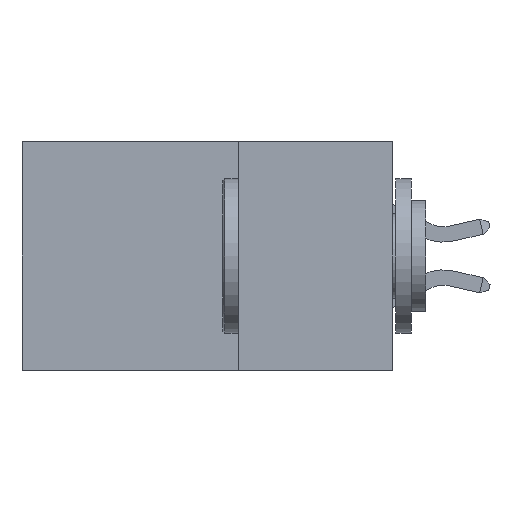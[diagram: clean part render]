
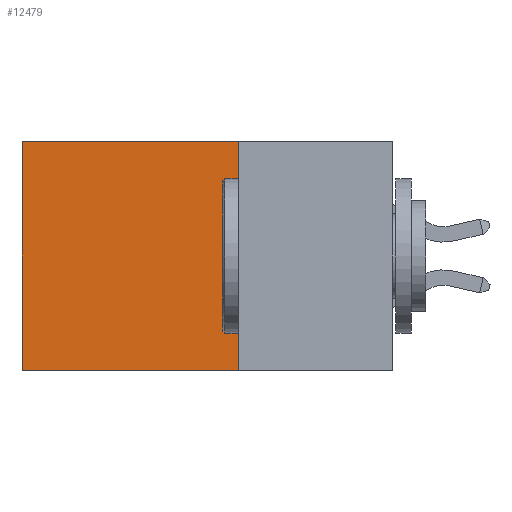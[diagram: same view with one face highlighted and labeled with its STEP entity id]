
A CAD part, left-side view. The second image highlights one B-rep face of the part: STEP entity #12479.
In plain terms, the highlighted planar face has unit normal (-1, 0, 0).
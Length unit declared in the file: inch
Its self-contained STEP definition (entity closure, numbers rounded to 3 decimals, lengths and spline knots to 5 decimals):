
#1397 = CARTESIAN_POINT ( 'NONE',  ( 0.2875, 0.6, 0. ) ) ;
#2869 = EDGE_CURVE ( 'NONE', #35021, #25414, #23550, .T. ) ;
#4264 = EDGE_CURVE ( 'NONE', #35021, #15242, #15848, .T. ) ;
#4286 = VECTOR ( 'NONE', #32611, 39.37008 ) ;
#5273 = CARTESIAN_POINT ( 'NONE',  ( 0.2875, 0.25, 0. ) ) ;
#5364 = DIRECTION ( 'NONE',  ( 0., 0., -1. ) ) ;
#6828 = CARTESIAN_POINT ( 'NONE',  ( 0.2875, 0.25, 0. ) ) ;
#7261 = DIRECTION ( 'NONE',  ( 0., 0., -1. ) ) ;
#8185 = CARTESIAN_POINT ( 'NONE',  ( 0.2875, 0.25, 0. ) ) ;
#8508 = DIRECTION ( 'NONE',  ( 0., 1., 0. ) ) ;
#10501 = VERTEX_POINT ( 'NONE', #10815 ) ;
#10815 = CARTESIAN_POINT ( 'NONE',  ( 0.2875, 0.6, -0.37 ) ) ;
#11684 = DIRECTION ( 'NONE',  ( 1., 0., 0. ) ) ;
#12479 = ADVANCED_FACE ( 'NONE', ( #28546 ), #18014, .F. ) ;
#15242 = VERTEX_POINT ( 'NONE', #37734 ) ;
#15775 = CARTESIAN_POINT ( 'NONE',  ( 0.2875, 0.25, 0. ) ) ;
#15848 = LINE ( 'NONE', #15775, #37010 ) ;
#16055 = EDGE_CURVE ( 'NONE', #25414, #10501, #39386, .T. ) ;
#18014 = PLANE ( 'NONE',  #30349 ) ;
#18202 = CARTESIAN_POINT ( 'NONE',  ( 0.2875, 0.6, 0. ) ) ;
#19300 = DIRECTION ( 'NONE',  ( 0., 0., -1. ) ) ;
#21228 = VECTOR ( 'NONE', #7261, 39.37008 ) ;
#23550 = LINE ( 'NONE', #5273, #28610 ) ;
#24911 = ORIENTED_EDGE ( 'NONE', *, *, #4264, .F. ) ;
#25414 = VERTEX_POINT ( 'NONE', #18202 ) ;
#26799 = EDGE_CURVE ( 'NONE', #15242, #10501, #33981, .T. ) ;
#26828 = ORIENTED_EDGE ( 'NONE', *, *, #26799, .F. ) ;
#27762 = ORIENTED_EDGE ( 'NONE', *, *, #16055, .T. ) ;
#28546 = FACE_OUTER_BOUND ( 'NONE', #32830, .T. ) ;
#28610 = VECTOR ( 'NONE', #8508, 39.37008 ) ;
#30349 = AXIS2_PLACEMENT_3D ( 'NONE', #8185, #11684, #5364 ) ;
#32611 = DIRECTION ( 'NONE',  ( 0., 1., 0. ) ) ;
#32830 = EDGE_LOOP ( 'NONE', ( #27762, #26828, #24911, #39132 ) ) ;
#33981 = LINE ( 'NONE', #39634, #4286 ) ;
#35021 = VERTEX_POINT ( 'NONE', #6828 ) ;
#37010 = VECTOR ( 'NONE', #19300, 39.37008 ) ;
#37734 = CARTESIAN_POINT ( 'NONE',  ( 0.2875, 0.25, -0.37 ) ) ;
#39132 = ORIENTED_EDGE ( 'NONE', *, *, #2869, .T. ) ;
#39386 = LINE ( 'NONE', #1397, #21228 ) ;
#39634 = CARTESIAN_POINT ( 'NONE',  ( 0.2875, 0.25, -0.37 ) ) ;
